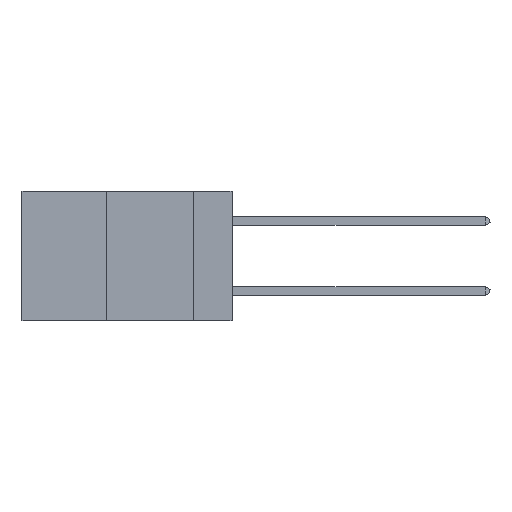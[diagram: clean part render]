
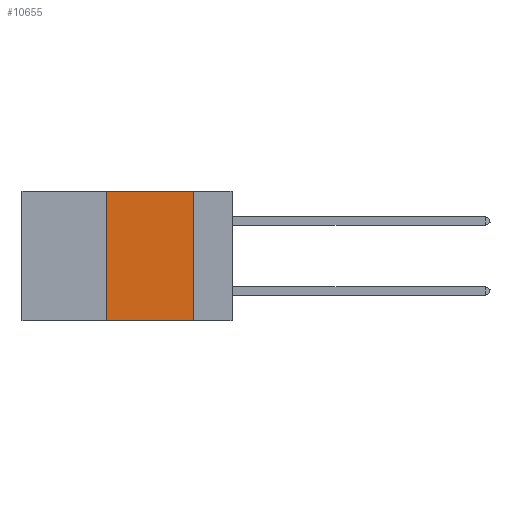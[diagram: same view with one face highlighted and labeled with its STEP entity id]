
A CAD part, left-side view. The second image highlights one B-rep face of the part: STEP entity #10655.
In plain terms, the highlighted planar face has unit normal (-1, 0, 0).
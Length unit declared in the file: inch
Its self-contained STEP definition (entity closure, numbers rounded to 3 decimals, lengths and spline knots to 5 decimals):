
#206 = EDGE_CURVE ( 'NONE', #3610, #3299, #10534, .T. ) ;
#398 = FACE_OUTER_BOUND ( 'NONE', #11864, .T. ) ;
#1187 = CARTESIAN_POINT ( 'NONE',  ( 0., 0.36, -0.37 ) ) ;
#2303 = VECTOR ( 'NONE', #4041, 39.37008 ) ;
#2337 = EDGE_CURVE ( 'NONE', #2406, #3610, #3201, .T. ) ;
#2406 = VERTEX_POINT ( 'NONE', #1187 ) ;
#3201 = LINE ( 'NONE', #4997, #2303 ) ;
#3299 = VERTEX_POINT ( 'NONE', #6391 ) ;
#3394 = VECTOR ( 'NONE', #6067, 39.37008 ) ;
#3399 = DIRECTION ( 'NONE',  ( 0., -1., 0. ) ) ;
#3596 = VERTEX_POINT ( 'NONE', #10312 ) ;
#3610 = VERTEX_POINT ( 'NONE', #4938 ) ;
#3623 = EDGE_CURVE ( 'NONE', #2406, #3596, #9190, .T. ) ;
#3709 = LINE ( 'NONE', #5124, #3394 ) ;
#3747 = EDGE_CURVE ( 'NONE', #3299, #3596, #3709, .T. ) ;
#3859 = DIRECTION ( 'NONE',  ( 1., 0., 0. ) ) ;
#4009 = DIRECTION ( 'NONE',  ( 0., -1., 0. ) ) ;
#4041 = DIRECTION ( 'NONE',  ( 0., 0., 1. ) ) ;
#4508 = CARTESIAN_POINT ( 'NONE',  ( 0., 0.6, 0. ) ) ;
#4894 = ORIENTED_EDGE ( 'NONE', *, *, #3747, .F. ) ;
#4938 = CARTESIAN_POINT ( 'NONE',  ( 0., 0.36, 0. ) ) ;
#4997 = CARTESIAN_POINT ( 'NONE',  ( 0., 0.36, 0. ) ) ;
#5124 = CARTESIAN_POINT ( 'NONE',  ( 0., 0.11, 0. ) ) ;
#5806 = VECTOR ( 'NONE', #3399, 39.37008 ) ;
#6067 = DIRECTION ( 'NONE',  ( 0., 0., -1. ) ) ;
#6391 = CARTESIAN_POINT ( 'NONE',  ( 0., 0.11, 0. ) ) ;
#6838 = VECTOR ( 'NONE', #4009, 39.37008 ) ;
#8448 = CARTESIAN_POINT ( 'NONE',  ( 0., 0.6, 0. ) ) ;
#9190 = LINE ( 'NONE', #10351, #6838 ) ;
#9357 = PLANE ( 'NONE',  #10749 ) ;
#9694 = ORIENTED_EDGE ( 'NONE', *, *, #206, .F. ) ;
#9960 = ORIENTED_EDGE ( 'NONE', *, *, #2337, .F. ) ;
#10226 = DIRECTION ( 'NONE',  ( 0., 0., -1. ) ) ;
#10245 = ORIENTED_EDGE ( 'NONE', *, *, #3623, .T. ) ;
#10312 = CARTESIAN_POINT ( 'NONE',  ( 0., 0.11, -0.37 ) ) ;
#10351 = CARTESIAN_POINT ( 'NONE',  ( 0., 0.6, -0.37 ) ) ;
#10534 = LINE ( 'NONE', #4508, #5806 ) ;
#10655 = ADVANCED_FACE ( 'NONE', ( #398 ), #9357, .F. ) ;
#10749 = AXIS2_PLACEMENT_3D ( 'NONE', #8448, #3859, #10226 ) ;
#11864 = EDGE_LOOP ( 'NONE', ( #4894, #9694, #9960, #10245 ) ) ;
